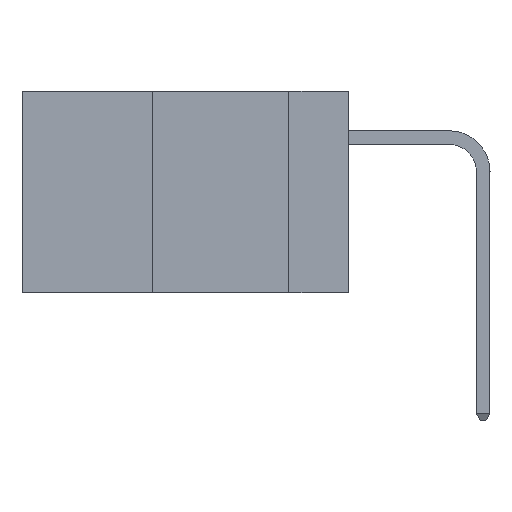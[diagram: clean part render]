
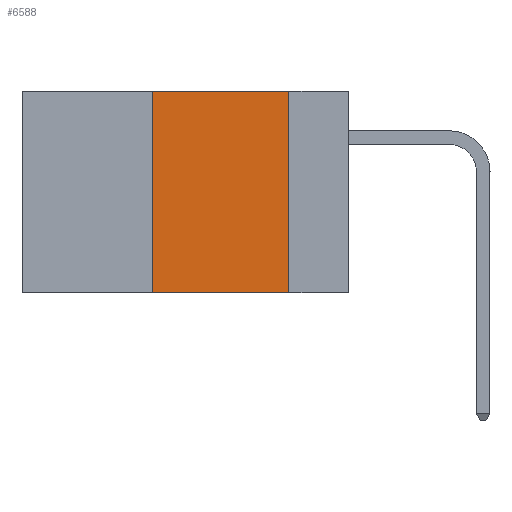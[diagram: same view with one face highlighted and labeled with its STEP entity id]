
A CAD part, left-side view. The second image highlights one B-rep face of the part: STEP entity #6588.
In plain terms, the highlighted planar face has unit normal (-1, 0, 0).
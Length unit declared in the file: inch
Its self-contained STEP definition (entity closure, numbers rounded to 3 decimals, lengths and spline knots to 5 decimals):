
#817 = ORIENTED_EDGE ( 'NONE', *, *, #17246, .T. ) ;
#902 = VERTEX_POINT ( 'NONE', #3081 ) ;
#1695 = CARTESIAN_POINT ( 'NONE',  ( 0., 0.6, 0. ) ) ;
#2732 = VERTEX_POINT ( 'NONE', #7185 ) ;
#3081 = CARTESIAN_POINT ( 'NONE',  ( 0., 0.11, -0.37 ) ) ;
#3258 = EDGE_LOOP ( 'NONE', ( #20685, #19811, #19000, #817 ) ) ;
#3519 = LINE ( 'NONE', #15006, #15259 ) ;
#4079 = LINE ( 'NONE', #15416, #12069 ) ;
#4932 = DIRECTION ( 'NONE',  ( 0., 0., -1. ) ) ;
#5681 = DIRECTION ( 'NONE',  ( 0., 0., -1. ) ) ;
#6588 = ADVANCED_FACE ( 'NONE', ( #13791 ), #11527, .F. ) ;
#6928 = VECTOR ( 'NONE', #18865, 39.37008 ) ;
#7185 = CARTESIAN_POINT ( 'NONE',  ( 0., 0.11, 0. ) ) ;
#8053 = EDGE_CURVE ( 'NONE', #23276, #17748, #3519, .T. ) ;
#9142 = DIRECTION ( 'NONE',  ( 0., 0., 1. ) ) ;
#9284 = LINE ( 'NONE', #20615, #13003 ) ;
#9610 = DIRECTION ( 'NONE',  ( 0., -1., 0. ) ) ;
#11527 = PLANE ( 'NONE',  #23372 ) ;
#12069 = VECTOR ( 'NONE', #9610, 39.37008 ) ;
#13003 = VECTOR ( 'NONE', #4932, 39.37008 ) ;
#13791 = FACE_OUTER_BOUND ( 'NONE', #3258, .T. ) ;
#15006 = CARTESIAN_POINT ( 'NONE',  ( 0., 0.36, 0. ) ) ;
#15259 = VECTOR ( 'NONE', #9142, 39.37008 ) ;
#15416 = CARTESIAN_POINT ( 'NONE',  ( 0., 0.6, 0. ) ) ;
#16404 = CARTESIAN_POINT ( 'NONE',  ( 0., 0.36, 0. ) ) ;
#17246 = EDGE_CURVE ( 'NONE', #23276, #902, #20825, .T. ) ;
#17343 = DIRECTION ( 'NONE',  ( 1., 0., 0. ) ) ;
#17748 = VERTEX_POINT ( 'NONE', #16404 ) ;
#18865 = DIRECTION ( 'NONE',  ( 0., -1., 0. ) ) ;
#19000 = ORIENTED_EDGE ( 'NONE', *, *, #8053, .F. ) ;
#19254 = CARTESIAN_POINT ( 'NONE',  ( 0., 0.36, -0.37 ) ) ;
#19811 = ORIENTED_EDGE ( 'NONE', *, *, #22094, .F. ) ;
#20615 = CARTESIAN_POINT ( 'NONE',  ( 0., 0.11, 0. ) ) ;
#20685 = ORIENTED_EDGE ( 'NONE', *, *, #23135, .F. ) ;
#20825 = LINE ( 'NONE', #22817, #6928 ) ;
#22094 = EDGE_CURVE ( 'NONE', #17748, #2732, #4079, .T. ) ;
#22817 = CARTESIAN_POINT ( 'NONE',  ( 0., 0.6, -0.37 ) ) ;
#23135 = EDGE_CURVE ( 'NONE', #2732, #902, #9284, .T. ) ;
#23276 = VERTEX_POINT ( 'NONE', #19254 ) ;
#23372 = AXIS2_PLACEMENT_3D ( 'NONE', #1695, #17343, #5681 ) ;
